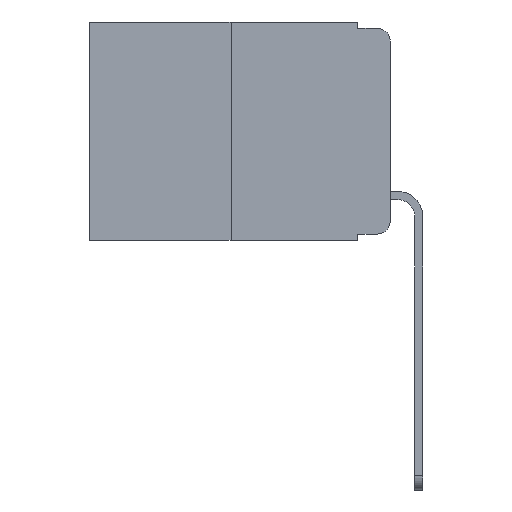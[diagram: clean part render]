
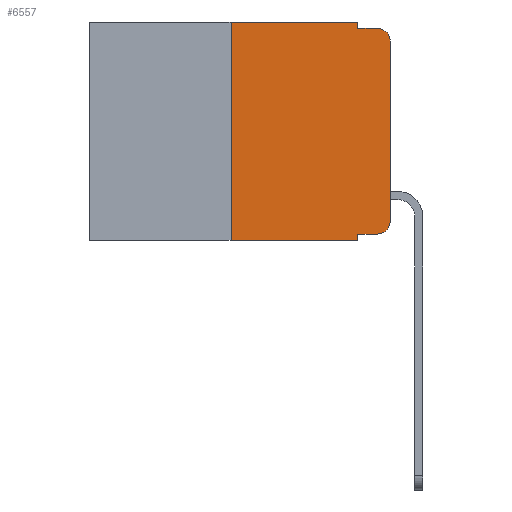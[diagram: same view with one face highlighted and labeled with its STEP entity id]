
A CAD part, left-side view. The second image highlights one B-rep face of the part: STEP entity #6557.
In plain terms, the highlighted planar face has unit normal (-1, 0, 0).
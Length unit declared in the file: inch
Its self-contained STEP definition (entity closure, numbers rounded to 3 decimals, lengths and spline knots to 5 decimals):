
#204 = VECTOR ( 'NONE', #9914, 39.37008 ) ;
#378 = ORIENTED_EDGE ( 'NONE', *, *, #3936, .F. ) ;
#568 = CARTESIAN_POINT ( 'NONE',  ( 0., 0.051, 0. ) ) ;
#634 = DIRECTION ( 'NONE',  ( 0., 0., -1. ) ) ;
#735 = DIRECTION ( 'NONE',  ( 0., -1., 0. ) ) ;
#837 = DIRECTION ( 'NONE',  ( 0., -1., 0. ) ) ;
#906 = CARTESIAN_POINT ( 'NONE',  ( 0., 0.473, 0. ) ) ;
#914 = VERTEX_POINT ( 'NONE', #13172 ) ;
#1815 = DIRECTION ( 'NONE',  ( 1., 0., 0. ) ) ;
#1852 = VERTEX_POINT ( 'NONE', #10170 ) ;
#2141 = DIRECTION ( 'NONE',  ( 0., 0., -1. ) ) ;
#2364 = AXIS2_PLACEMENT_3D ( 'NONE', #14189, #7343, #15317 ) ;
#2398 = CARTESIAN_POINT ( 'NONE',  ( 0., 0., 0. ) ) ;
#2526 = VERTEX_POINT ( 'NONE', #3349 ) ;
#2735 = DIRECTION ( 'NONE',  ( -1., 0., 0. ) ) ;
#2762 = CARTESIAN_POINT ( 'NONE',  ( 0., 0.051, -0.01 ) ) ;
#2808 = VERTEX_POINT ( 'NONE', #2762 ) ;
#3172 = LINE ( 'NONE', #4958, #9329 ) ;
#3349 = CARTESIAN_POINT ( 'NONE',  ( 0., 0., -0.313 ) ) ;
#3438 = CARTESIAN_POINT ( 'NONE',  ( 0., 0.25, 0. ) ) ;
#3511 = EDGE_CURVE ( 'NONE', #13289, #6694, #12896, .T. ) ;
#3614 = LINE ( 'NONE', #7395, #6585 ) ;
#3731 = ORIENTED_EDGE ( 'NONE', *, *, #4306, .F. ) ;
#3911 = EDGE_CURVE ( 'NONE', #11228, #2526, #9692, .T. ) ;
#3914 = EDGE_CURVE ( 'NONE', #1852, #11228, #7312, .T. ) ;
#3915 = EDGE_CURVE ( 'NONE', #1852, #6694, #13047, .T. ) ;
#3936 = EDGE_CURVE ( 'NONE', #13289, #10828, #3614, .T. ) ;
#3937 = EDGE_CURVE ( 'NONE', #10426, #2808, #3172, .T. ) ;
#4306 = EDGE_CURVE ( 'NONE', #2808, #14922, #13563, .T. ) ;
#4324 = EDGE_CURVE ( 'NONE', #10828, #10426, #12858, .T. ) ;
#4387 = EDGE_CURVE ( 'NONE', #914, #14922, #14426, .T. ) ;
#4526 = EDGE_CURVE ( 'NONE', #2526, #914, #8926, .T. ) ;
#4958 = CARTESIAN_POINT ( 'NONE',  ( 0., 0.051, 0. ) ) ;
#5154 = CARTESIAN_POINT ( 'NONE',  ( 0., 0.051, -0.01 ) ) ;
#5418 = FACE_OUTER_BOUND ( 'NONE', #9768, .T. ) ;
#5703 = CARTESIAN_POINT ( 'NONE',  ( 0., 0.25, -0.343 ) ) ;
#6160 = CARTESIAN_POINT ( 'NONE',  ( 0., 0.051, -0.333 ) ) ;
#6557 = ADVANCED_FACE ( 'NONE', ( #5418 ), #9437, .F. ) ;
#6585 = VECTOR ( 'NONE', #8557, 39.37008 ) ;
#6619 = CARTESIAN_POINT ( 'NONE',  ( 0., 0.02, -0.01 ) ) ;
#6694 = VERTEX_POINT ( 'NONE', #15268 ) ;
#7312 = LINE ( 'NONE', #6160, #15684 ) ;
#7343 = DIRECTION ( 'NONE',  ( -1., 0., 0. ) ) ;
#7395 = CARTESIAN_POINT ( 'NONE',  ( 0., 0.25, 0. ) ) ;
#7966 = ORIENTED_EDGE ( 'NONE', *, *, #3511, .T. ) ;
#8266 = CARTESIAN_POINT ( 'NONE',  ( 0., 0.473, 0. ) ) ;
#8557 = DIRECTION ( 'NONE',  ( 0., 0., 1. ) ) ;
#8621 = CARTESIAN_POINT ( 'NONE',  ( 0., 0.473, -0.343 ) ) ;
#8926 = LINE ( 'NONE', #2398, #14246 ) ;
#8941 = CARTESIAN_POINT ( 'NONE',  ( 0., 0.02, -0.333 ) ) ;
#9329 = VECTOR ( 'NONE', #634, 39.37008 ) ;
#9437 = PLANE ( 'NONE',  #13424 ) ;
#9675 = VECTOR ( 'NONE', #2141, 39.37008 ) ;
#9692 = CIRCLE ( 'NONE', #2364, 0.02 ) ;
#9768 = EDGE_LOOP ( 'NONE', ( #15953, #11722, #3731, #10492, #15261, #378, #7966, #11736, #10142, #13877 ) ) ;
#9871 = DIRECTION ( 'NONE',  ( 0., 0., 1. ) ) ;
#9914 = DIRECTION ( 'NONE',  ( 0., -1., 0. ) ) ;
#10115 = CARTESIAN_POINT ( 'NONE',  ( 0., 0.02, -0.03 ) ) ;
#10142 = ORIENTED_EDGE ( 'NONE', *, *, #3914, .T. ) ;
#10170 = CARTESIAN_POINT ( 'NONE',  ( 0., 0.051, -0.333 ) ) ;
#10240 = VECTOR ( 'NONE', #735, 39.37008 ) ;
#10426 = VERTEX_POINT ( 'NONE', #13479 ) ;
#10492 = ORIENTED_EDGE ( 'NONE', *, *, #3937, .F. ) ;
#10576 = DIRECTION ( 'NONE',  ( 0., 0., -1. ) ) ;
#10773 = DIRECTION ( 'NONE',  ( 0., -1., 0. ) ) ;
#10828 = VERTEX_POINT ( 'NONE', #3438 ) ;
#11228 = VERTEX_POINT ( 'NONE', #8941 ) ;
#11263 = DIRECTION ( 'NONE',  ( 0., 0., -1. ) ) ;
#11618 = AXIS2_PLACEMENT_3D ( 'NONE', #10115, #2735, #11263 ) ;
#11722 = ORIENTED_EDGE ( 'NONE', *, *, #4387, .T. ) ;
#11736 = ORIENTED_EDGE ( 'NONE', *, *, #3915, .F. ) ;
#12858 = LINE ( 'NONE', #906, #204 ) ;
#12896 = LINE ( 'NONE', #8621, #10240 ) ;
#13047 = LINE ( 'NONE', #568, #9675 ) ;
#13172 = CARTESIAN_POINT ( 'NONE',  ( 0., 0., -0.03 ) ) ;
#13200 = VECTOR ( 'NONE', #837, 39.37008 ) ;
#13289 = VERTEX_POINT ( 'NONE', #5703 ) ;
#13424 = AXIS2_PLACEMENT_3D ( 'NONE', #8266, #1815, #10576 ) ;
#13479 = CARTESIAN_POINT ( 'NONE',  ( 0., 0.051, 0. ) ) ;
#13563 = LINE ( 'NONE', #5154, #13200 ) ;
#13877 = ORIENTED_EDGE ( 'NONE', *, *, #3911, .T. ) ;
#14189 = CARTESIAN_POINT ( 'NONE',  ( 0., 0.02, -0.313 ) ) ;
#14246 = VECTOR ( 'NONE', #9871, 39.37008 ) ;
#14426 = CIRCLE ( 'NONE', #11618, 0.02 ) ;
#14922 = VERTEX_POINT ( 'NONE', #6619 ) ;
#15261 = ORIENTED_EDGE ( 'NONE', *, *, #4324, .F. ) ;
#15268 = CARTESIAN_POINT ( 'NONE',  ( 0., 0.051, -0.343 ) ) ;
#15317 = DIRECTION ( 'NONE',  ( 0., 0., -1. ) ) ;
#15684 = VECTOR ( 'NONE', #10773, 39.37008 ) ;
#15953 = ORIENTED_EDGE ( 'NONE', *, *, #4526, .T. ) ;
